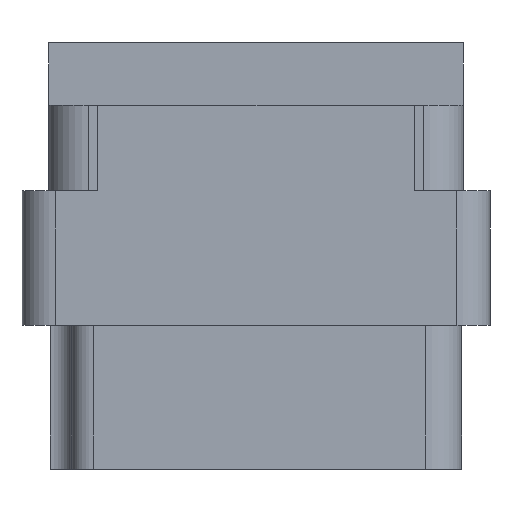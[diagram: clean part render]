
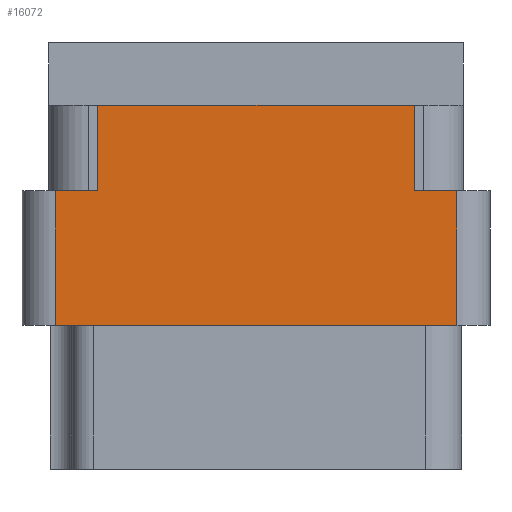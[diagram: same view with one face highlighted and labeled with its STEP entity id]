
A CAD part, left-side view. The second image highlights one B-rep face of the part: STEP entity #16072.
In plain terms, the highlighted planar face has unit normal (-1, 0, 0).
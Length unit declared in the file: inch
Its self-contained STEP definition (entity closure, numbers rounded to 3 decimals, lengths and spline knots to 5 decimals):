
#64 = LINE ( 'NONE', #7379, #15249 ) ;
#913 = EDGE_CURVE ( 'NONE', #34254, #30252, #15929, .T. ) ;
#1333 = VECTOR ( 'NONE', #11302, 39.37008 ) ;
#1719 = DIRECTION ( 'NONE',  ( 0., -1., 0. ) ) ;
#2083 = DIRECTION ( 'NONE',  ( 0., 1., 0. ) ) ;
#4457 = VECTOR ( 'NONE', #2083, 39.37008 ) ;
#4798 = CARTESIAN_POINT ( 'NONE',  ( -1.296, -0.376, -0.798 ) ) ;
#4973 = VERTEX_POINT ( 'NONE', #28431 ) ;
#5457 = DIRECTION ( 'NONE',  ( -1., 0., 0. ) ) ;
#5510 = LINE ( 'NONE', #8632, #24654 ) ;
#5648 = CARTESIAN_POINT ( 'NONE',  ( -1.296, -0.376, -0.529 ) ) ;
#5710 = DIRECTION ( 'NONE',  ( 0., 0., -1. ) ) ;
#5832 = VERTEX_POINT ( 'NONE', #13532 ) ;
#7201 = ORIENTED_EDGE ( 'NONE', *, *, #11516, .T. ) ;
#7379 = CARTESIAN_POINT ( 'NONE',  ( -1.296, 0.438, -0.117 ) ) ;
#7481 = LINE ( 'NONE', #41758, #12539 ) ;
#7993 = CARTESIAN_POINT ( 'NONE',  ( -1.296, 0.296, -0.277 ) ) ;
#8206 = EDGE_CURVE ( 'NONE', #11898, #4973, #42792, .T. ) ;
#8391 = DIRECTION ( 'NONE',  ( 0., 0., 1. ) ) ;
#8632 = CARTESIAN_POINT ( 'NONE',  ( -1.296, 0., -0.277 ) ) ;
#8797 = VERTEX_POINT ( 'NONE', #45999 ) ;
#9334 = CARTESIAN_POINT ( 'NONE',  ( -1.296, 0., -0.529 ) ) ;
#10752 = CARTESIAN_POINT ( 'NONE',  ( -1.296, -0.296, -0.117 ) ) ;
#11302 = DIRECTION ( 'NONE',  ( 0., 0., 1. ) ) ;
#11384 = ORIENTED_EDGE ( 'NONE', *, *, #8206, .F. ) ;
#11516 = EDGE_CURVE ( 'NONE', #5832, #23612, #7481, .T. ) ;
#11898 = VERTEX_POINT ( 'NONE', #5648 ) ;
#12539 = VECTOR ( 'NONE', #34638, 39.37008 ) ;
#13214 = LINE ( 'NONE', #4798, #17685 ) ;
#13532 = CARTESIAN_POINT ( 'NONE',  ( -1.296, -0.296, -0.277 ) ) ;
#14452 = DIRECTION ( 'NONE',  ( 0., -1., 0. ) ) ;
#15249 = VECTOR ( 'NONE', #14452, 39.37008 ) ;
#15929 = LINE ( 'NONE', #7993, #1333 ) ;
#16072 = ADVANCED_FACE ( 'NONE', ( #38154 ), #37872, .T. ) ;
#16564 = DIRECTION ( 'NONE',  ( 0., -1., 0. ) ) ;
#17685 = VECTOR ( 'NONE', #8391, 39.37008 ) ;
#17823 = ORIENTED_EDGE ( 'NONE', *, *, #31507, .F. ) ;
#18197 = EDGE_CURVE ( 'NONE', #8797, #34254, #5510, .T. ) ;
#20216 = ORIENTED_EDGE ( 'NONE', *, *, #38090, .T. ) ;
#20533 = ORIENTED_EDGE ( 'NONE', *, *, #913, .F. ) ;
#23612 = VERTEX_POINT ( 'NONE', #10752 ) ;
#23949 = CARTESIAN_POINT ( 'NONE',  ( -1.296, 0., -0.277 ) ) ;
#24575 = EDGE_CURVE ( 'NONE', #11898, #38735, #13214, .T. ) ;
#24654 = VECTOR ( 'NONE', #1719, 39.37008 ) ;
#24656 = CARTESIAN_POINT ( 'NONE',  ( -1.296, 0.296, -0.277 ) ) ;
#26420 = EDGE_CURVE ( 'NONE', #5832, #38735, #43523, .T. ) ;
#27003 = CARTESIAN_POINT ( 'NONE',  ( -1.296, -0.438, -0.798 ) ) ;
#27260 = CARTESIAN_POINT ( 'NONE',  ( -1.296, 0.376, -0.798 ) ) ;
#28431 = CARTESIAN_POINT ( 'NONE',  ( -1.296, 0.376, -0.529 ) ) ;
#30252 = VERTEX_POINT ( 'NONE', #33316 ) ;
#31507 = EDGE_CURVE ( 'NONE', #30252, #23612, #64, .T. ) ;
#32628 = AXIS2_PLACEMENT_3D ( 'NONE', #27003, #5457, #41038 ) ;
#32870 = ORIENTED_EDGE ( 'NONE', *, *, #24575, .T. ) ;
#33316 = CARTESIAN_POINT ( 'NONE',  ( -1.296, 0.296, -0.117 ) ) ;
#33994 = ORIENTED_EDGE ( 'NONE', *, *, #26420, .F. ) ;
#34254 = VERTEX_POINT ( 'NONE', #24656 ) ;
#34638 = DIRECTION ( 'NONE',  ( 0., 0., 1. ) ) ;
#37872 = PLANE ( 'NONE',  #32628 ) ;
#38090 = EDGE_CURVE ( 'NONE', #8797, #4973, #43817, .T. ) ;
#38154 = FACE_OUTER_BOUND ( 'NONE', #43794, .T. ) ;
#38735 = VERTEX_POINT ( 'NONE', #42663 ) ;
#40860 = ORIENTED_EDGE ( 'NONE', *, *, #18197, .F. ) ;
#41038 = DIRECTION ( 'NONE',  ( 0., 0., 1. ) ) ;
#41758 = CARTESIAN_POINT ( 'NONE',  ( -1.296, -0.296, -0.277 ) ) ;
#42149 = VECTOR ( 'NONE', #5710, 39.37008 ) ;
#42663 = CARTESIAN_POINT ( 'NONE',  ( -1.296, -0.376, -0.277 ) ) ;
#42792 = LINE ( 'NONE', #9334, #4457 ) ;
#42994 = VECTOR ( 'NONE', #16564, 39.37008 ) ;
#43523 = LINE ( 'NONE', #23949, #42994 ) ;
#43794 = EDGE_LOOP ( 'NONE', ( #40860, #20216, #11384, #32870, #33994, #7201, #17823, #20533 ) ) ;
#43817 = LINE ( 'NONE', #27260, #42149 ) ;
#45999 = CARTESIAN_POINT ( 'NONE',  ( -1.296, 0.376, -0.277 ) ) ;
